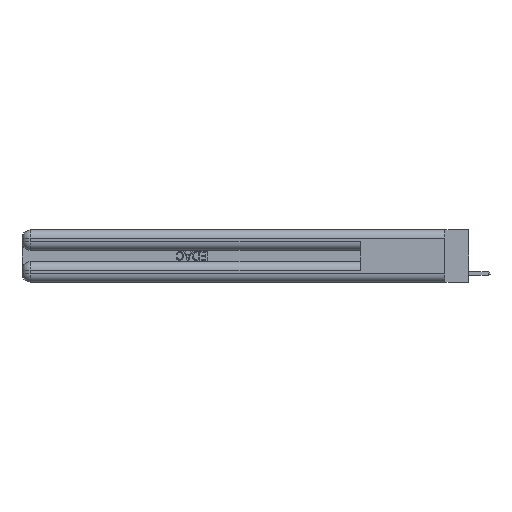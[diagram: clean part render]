
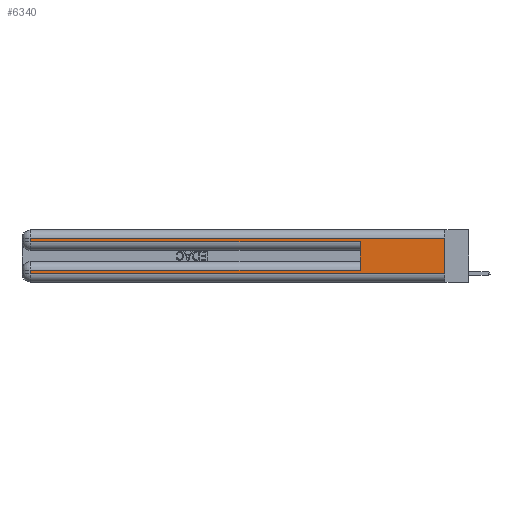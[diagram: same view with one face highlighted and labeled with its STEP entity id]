
A CAD part, left-side view. The second image highlights one B-rep face of the part: STEP entity #6340.
In plain terms, the highlighted planar face has unit normal (-1, 0, 0).
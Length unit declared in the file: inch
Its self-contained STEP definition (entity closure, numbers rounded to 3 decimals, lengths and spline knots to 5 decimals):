
#583 = VERTEX_POINT ( 'NONE', #21399 ) ;
#764 = VERTEX_POINT ( 'NONE', #24304 ) ;
#1352 = VECTOR ( 'NONE', #18801, 39.37008 ) ;
#1474 = DIRECTION ( 'NONE',  ( 0., -1., 0. ) ) ;
#1957 = VECTOR ( 'NONE', #28687, 39.37008 ) ;
#2712 = CARTESIAN_POINT ( 'NONE',  ( 0., 0., 0.31 ) ) ;
#3838 = CARTESIAN_POINT ( 'NONE',  ( 0., 0., 0.31 ) ) ;
#4043 = VERTEX_POINT ( 'NONE', #7121 ) ;
#4106 = CARTESIAN_POINT ( 'NONE',  ( 0., 0., 0.37 ) ) ;
#4402 = DIRECTION ( 'NONE',  ( 0., 0., -1. ) ) ;
#4411 = EDGE_CURVE ( 'NONE', #10799, #9664, #5050, .T. ) ;
#4466 = EDGE_CURVE ( 'NONE', #9664, #21949, #4889, .T. ) ;
#4889 = LINE ( 'NONE', #23617, #20614 ) ;
#5050 = LINE ( 'NONE', #2712, #1957 ) ;
#6080 = CARTESIAN_POINT ( 'NONE',  ( 0., 0.6, 0.085 ) ) ;
#6340 = ADVANCED_FACE ( 'NONE', ( #22189 ), #24498, .F. ) ;
#6717 = ORIENTED_EDGE ( 'NONE', *, *, #18217, .F. ) ;
#6788 = LINE ( 'NONE', #27963, #17536 ) ;
#7121 = CARTESIAN_POINT ( 'NONE',  ( 0., 2.94, 0.085 ) ) ;
#7502 = DIRECTION ( 'NONE',  ( 0., 0., -1. ) ) ;
#7531 = AXIS2_PLACEMENT_3D ( 'NONE', #17577, #24793, #10523 ) ;
#8246 = CARTESIAN_POINT ( 'NONE',  ( 0., 0., 0.285 ) ) ;
#8340 = ORIENTED_EDGE ( 'NONE', *, *, #4411, .T. ) ;
#9439 = CARTESIAN_POINT ( 'NONE',  ( 0., 0., 0.06 ) ) ;
#9664 = VERTEX_POINT ( 'NONE', #24571 ) ;
#10523 = DIRECTION ( 'NONE',  ( 0., 0., -1. ) ) ;
#10799 = VERTEX_POINT ( 'NONE', #3838 ) ;
#11476 = VERTEX_POINT ( 'NONE', #6080 ) ;
#11648 = ORIENTED_EDGE ( 'NONE', *, *, #12821, .T. ) ;
#12000 = VECTOR ( 'NONE', #1474, 39.37008 ) ;
#12292 = ORIENTED_EDGE ( 'NONE', *, *, #4466, .T. ) ;
#12335 = VERTEX_POINT ( 'NONE', #28605 ) ;
#12821 = EDGE_CURVE ( 'NONE', #11476, #4043, #20231, .T. ) ;
#13597 = DIRECTION ( 'NONE',  ( 0., 1., 0. ) ) ;
#14282 = DIRECTION ( 'NONE',  ( 0., 0., 1. ) ) ;
#14965 = EDGE_CURVE ( 'NONE', #21949, #12335, #20234, .T. ) ;
#16134 = DIRECTION ( 'NONE',  ( 0., 0., -1. ) ) ;
#16186 = LINE ( 'NONE', #9439, #1352 ) ;
#16222 = LINE ( 'NONE', #4106, #16488 ) ;
#16488 = VECTOR ( 'NONE', #4402, 39.37008 ) ;
#16946 = ORIENTED_EDGE ( 'NONE', *, *, #14965, .T. ) ;
#17324 = EDGE_CURVE ( 'NONE', #11476, #12335, #28724, .T. ) ;
#17536 = VECTOR ( 'NONE', #16134, 39.37008 ) ;
#17577 = CARTESIAN_POINT ( 'NONE',  ( 0., 0., 0.37 ) ) ;
#18217 = EDGE_CURVE ( 'NONE', #10799, #764, #16222, .T. ) ;
#18552 = CARTESIAN_POINT ( 'NONE',  ( 0., 2.94, 0.285 ) ) ;
#18801 = DIRECTION ( 'NONE',  ( 0., -1., 0. ) ) ;
#19341 = CARTESIAN_POINT ( 'NONE',  ( 0., 0.6, 0.145 ) ) ;
#19694 = EDGE_CURVE ( 'NONE', #583, #764, #16186, .T. ) ;
#19752 = ORIENTED_EDGE ( 'NONE', *, *, #17324, .F. ) ;
#20231 = LINE ( 'NONE', #22513, #21649 ) ;
#20234 = LINE ( 'NONE', #8246, #12000 ) ;
#20421 = ORIENTED_EDGE ( 'NONE', *, *, #19694, .T. ) ;
#20614 = VECTOR ( 'NONE', #7502, 39.37008 ) ;
#21399 = CARTESIAN_POINT ( 'NONE',  ( 0., 2.94, 0.06 ) ) ;
#21649 = VECTOR ( 'NONE', #13597, 39.37008 ) ;
#21837 = EDGE_LOOP ( 'NONE', ( #6717, #8340, #12292, #16946, #19752, #11648, #26731, #20421 ) ) ;
#21949 = VERTEX_POINT ( 'NONE', #18552 ) ;
#22189 = FACE_OUTER_BOUND ( 'NONE', #21837, .T. ) ;
#22513 = CARTESIAN_POINT ( 'NONE',  ( 0., 0., 0.085 ) ) ;
#23617 = CARTESIAN_POINT ( 'NONE',  ( 0., 2.94, 0.37 ) ) ;
#23881 = VECTOR ( 'NONE', #14282, 39.37008 ) ;
#24304 = CARTESIAN_POINT ( 'NONE',  ( 0., 0., 0.06 ) ) ;
#24498 = PLANE ( 'NONE',  #7531 ) ;
#24571 = CARTESIAN_POINT ( 'NONE',  ( 0., 2.94, 0.31 ) ) ;
#24793 = DIRECTION ( 'NONE',  ( 1., 0., 0. ) ) ;
#26731 = ORIENTED_EDGE ( 'NONE', *, *, #29556, .T. ) ;
#27963 = CARTESIAN_POINT ( 'NONE',  ( 0., 2.94, 0.37 ) ) ;
#28605 = CARTESIAN_POINT ( 'NONE',  ( 0., 0.6, 0.285 ) ) ;
#28687 = DIRECTION ( 'NONE',  ( 0., 1., 0. ) ) ;
#28724 = LINE ( 'NONE', #19341, #23881 ) ;
#29556 = EDGE_CURVE ( 'NONE', #4043, #583, #6788, .T. ) ;
